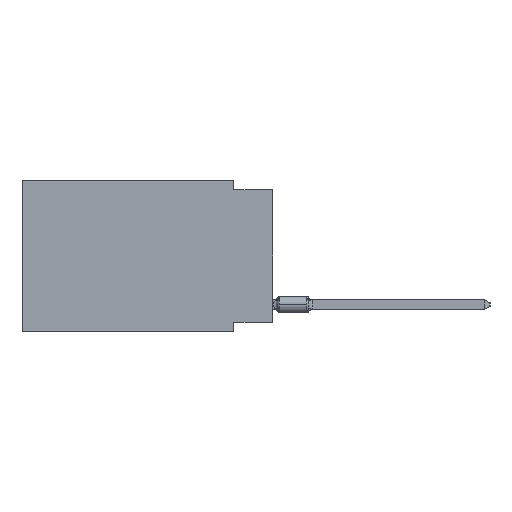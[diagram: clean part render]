
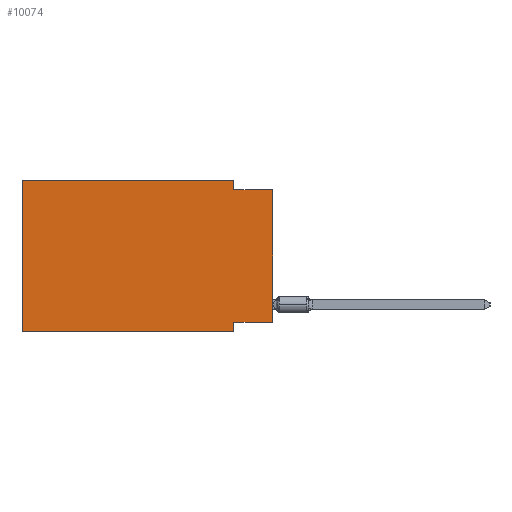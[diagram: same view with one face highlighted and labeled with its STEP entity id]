
A CAD part, left-side view. The second image highlights one B-rep face of the part: STEP entity #10074.
In plain terms, the highlighted planar face has unit normal (-1, 0, 0).
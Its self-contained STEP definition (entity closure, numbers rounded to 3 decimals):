
#83 = VECTOR ( 'NONE', #10268, 1000. ) ;
#583 = CARTESIAN_POINT ( 'NONE',  ( 0., 0., -9.271 ) ) ;
#1166 = EDGE_CURVE ( 'NONE', #20618, #7734, #22144, .T. ) ;
#1814 = LINE ( 'NONE', #7152, #15108 ) ;
#2322 = CARTESIAN_POINT ( 'NONE',  ( 0., 16.383, 0. ) ) ;
#2468 = DIRECTION ( 'NONE',  ( 0., -1., 0. ) ) ;
#2693 = LINE ( 'NONE', #20005, #12604 ) ;
#2965 = CARTESIAN_POINT ( 'NONE',  ( 0., 16.383, 0. ) ) ;
#3547 = PLANE ( 'NONE',  #7020 ) ;
#4609 = CARTESIAN_POINT ( 'NONE',  ( 0., 0., -9.271 ) ) ;
#5047 = LINE ( 'NONE', #19931, #31791 ) ;
#6150 = EDGE_CURVE ( 'NONE', #22469, #7734, #5047, .T. ) ;
#6889 = EDGE_CURVE ( 'NONE', #26168, #15097, #7366, .T. ) ;
#6952 = CARTESIAN_POINT ( 'NONE',  ( 0., 2.54, -9.906 ) ) ;
#7020 = AXIS2_PLACEMENT_3D ( 'NONE', #16448, #30706, #23754 ) ;
#7152 = CARTESIAN_POINT ( 'NONE',  ( 0., 0., -0.635 ) ) ;
#7366 = LINE ( 'NONE', #27079, #22353 ) ;
#7734 = VERTEX_POINT ( 'NONE', #18939 ) ;
#7969 = LINE ( 'NONE', #2965, #28854 ) ;
#10074 = ADVANCED_FACE ( 'NONE', ( #28573 ), #3547, .F. ) ;
#10268 = DIRECTION ( 'NONE',  ( 0., 1., 0. ) ) ;
#11428 = EDGE_LOOP ( 'NONE', ( #23208, #18396, #22623, #24113, #19155, #30547, #24926, #28450 ) ) ;
#11971 = DIRECTION ( 'NONE',  ( 0., -1., 0. ) ) ;
#12516 = DIRECTION ( 'NONE',  ( 0., 0., 1. ) ) ;
#12604 = VECTOR ( 'NONE', #15464, 1000. ) ;
#13181 = VECTOR ( 'NONE', #26976, 1000. ) ;
#13615 = VECTOR ( 'NONE', #19171, 1000. ) ;
#14101 = EDGE_CURVE ( 'NONE', #24295, #20727, #7969, .T. ) ;
#15097 = VERTEX_POINT ( 'NONE', #18078 ) ;
#15108 = VECTOR ( 'NONE', #11971, 1000. ) ;
#15464 = DIRECTION ( 'NONE',  ( 0., 0., 1. ) ) ;
#16448 = CARTESIAN_POINT ( 'NONE',  ( 0., 16.383, 0. ) ) ;
#16484 = EDGE_CURVE ( 'NONE', #23899, #15097, #1814, .T. ) ;
#18078 = CARTESIAN_POINT ( 'NONE',  ( 0., 0., -0.635 ) ) ;
#18157 = DIRECTION ( 'NONE',  ( 0., -1., 0. ) ) ;
#18396 = ORIENTED_EDGE ( 'NONE', *, *, #16484, .F. ) ;
#18544 = CARTESIAN_POINT ( 'NONE',  ( 0., 2.54, -9.271 ) ) ;
#18939 = CARTESIAN_POINT ( 'NONE',  ( 0., 2.54, -9.906 ) ) ;
#19155 = ORIENTED_EDGE ( 'NONE', *, *, #20126, .F. ) ;
#19171 = DIRECTION ( 'NONE',  ( 0., 0., -1. ) ) ;
#19658 = LINE ( 'NONE', #31777, #13615 ) ;
#19931 = CARTESIAN_POINT ( 'NONE',  ( 0., 16.383, -9.906 ) ) ;
#19988 = LINE ( 'NONE', #4609, #83 ) ;
#20005 = CARTESIAN_POINT ( 'NONE',  ( 0., 16.383, 0. ) ) ;
#20066 = CARTESIAN_POINT ( 'NONE',  ( 0., 2.54, -0.635 ) ) ;
#20126 = EDGE_CURVE ( 'NONE', #22469, #24295, #2693, .T. ) ;
#20618 = VERTEX_POINT ( 'NONE', #18544 ) ;
#20727 = VERTEX_POINT ( 'NONE', #26439 ) ;
#22144 = LINE ( 'NONE', #6952, #13181 ) ;
#22353 = VECTOR ( 'NONE', #12516, 1000. ) ;
#22469 = VERTEX_POINT ( 'NONE', #26804 ) ;
#22623 = ORIENTED_EDGE ( 'NONE', *, *, #30579, .F. ) ;
#23208 = ORIENTED_EDGE ( 'NONE', *, *, #6889, .T. ) ;
#23754 = DIRECTION ( 'NONE',  ( 0., 0., -1. ) ) ;
#23899 = VERTEX_POINT ( 'NONE', #20066 ) ;
#24113 = ORIENTED_EDGE ( 'NONE', *, *, #14101, .F. ) ;
#24295 = VERTEX_POINT ( 'NONE', #2322 ) ;
#24926 = ORIENTED_EDGE ( 'NONE', *, *, #1166, .F. ) ;
#25167 = EDGE_CURVE ( 'NONE', #26168, #20618, #19988, .T. ) ;
#26168 = VERTEX_POINT ( 'NONE', #583 ) ;
#26439 = CARTESIAN_POINT ( 'NONE',  ( 0., 2.54, 0. ) ) ;
#26804 = CARTESIAN_POINT ( 'NONE',  ( 0., 16.383, -9.906 ) ) ;
#26976 = DIRECTION ( 'NONE',  ( 0., 0., -1. ) ) ;
#27079 = CARTESIAN_POINT ( 'NONE',  ( 0., 0., 0. ) ) ;
#28450 = ORIENTED_EDGE ( 'NONE', *, *, #25167, .F. ) ;
#28573 = FACE_OUTER_BOUND ( 'NONE', #11428, .T. ) ;
#28854 = VECTOR ( 'NONE', #18157, 1000. ) ;
#30547 = ORIENTED_EDGE ( 'NONE', *, *, #6150, .T. ) ;
#30579 = EDGE_CURVE ( 'NONE', #20727, #23899, #19658, .T. ) ;
#30706 = DIRECTION ( 'NONE',  ( 1., 0., 0. ) ) ;
#31777 = CARTESIAN_POINT ( 'NONE',  ( 0., 2.54, 0. ) ) ;
#31791 = VECTOR ( 'NONE', #2468, 1000. ) ;
